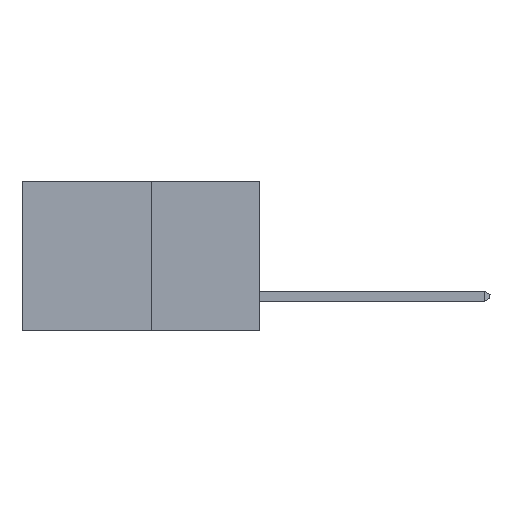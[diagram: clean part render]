
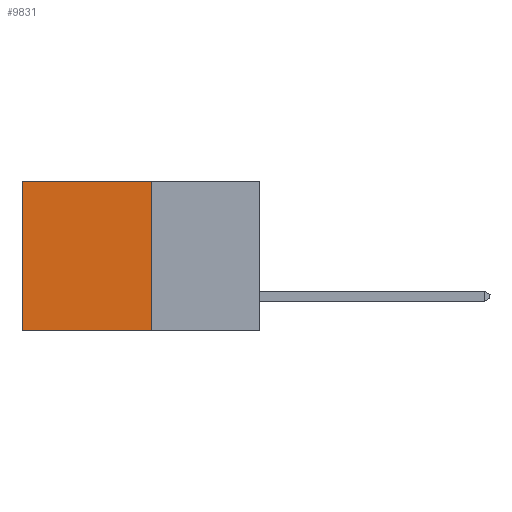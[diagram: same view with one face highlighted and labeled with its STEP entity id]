
A CAD part, left-side view. The second image highlights one B-rep face of the part: STEP entity #9831.
In plain terms, the highlighted planar face has unit normal (-1, 0, 0).
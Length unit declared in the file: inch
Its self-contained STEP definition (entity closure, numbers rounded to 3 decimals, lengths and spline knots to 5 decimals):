
#175 = PLANE ( 'NONE',  #7219 ) ;
#224 = EDGE_CURVE ( 'NONE', #5719, #2187, #7277, .T. ) ;
#442 = EDGE_CURVE ( 'NONE', #2187, #12836, #11072, .T. ) ;
#1648 = CARTESIAN_POINT ( 'NONE',  ( 0.277, 0.59, 0. ) ) ;
#1807 = EDGE_CURVE ( 'NONE', #11247, #12836, #8447, .T. ) ;
#2187 = VERTEX_POINT ( 'NONE', #1648 ) ;
#2620 = DIRECTION ( 'NONE',  ( 0., 0., -1. ) ) ;
#2775 = DIRECTION ( 'NONE',  ( 0., 0., -1. ) ) ;
#2966 = EDGE_CURVE ( 'NONE', #5719, #11247, #7939, .T. ) ;
#4893 = CARTESIAN_POINT ( 'NONE',  ( 0.277, 0.27, 0. ) ) ;
#5219 = DIRECTION ( 'NONE',  ( 0., 1., 0. ) ) ;
#5719 = VERTEX_POINT ( 'NONE', #4893 ) ;
#5843 = CARTESIAN_POINT ( 'NONE',  ( 0.277, 0.27, -0.37 ) ) ;
#6301 = FACE_OUTER_BOUND ( 'NONE', #10616, .T. ) ;
#6534 = ORIENTED_EDGE ( 'NONE', *, *, #1807, .F. ) ;
#6781 = DIRECTION ( 'NONE',  ( 0., 0., -1. ) ) ;
#7014 = CARTESIAN_POINT ( 'NONE',  ( 0.277, 0.27, -0.37 ) ) ;
#7073 = ORIENTED_EDGE ( 'NONE', *, *, #2966, .F. ) ;
#7118 = ORIENTED_EDGE ( 'NONE', *, *, #224, .T. ) ;
#7219 = AXIS2_PLACEMENT_3D ( 'NONE', #8006, #8978, #2620 ) ;
#7277 = LINE ( 'NONE', #9451, #11656 ) ;
#7328 = ORIENTED_EDGE ( 'NONE', *, *, #442, .T. ) ;
#7939 = LINE ( 'NONE', #7014, #12591 ) ;
#8006 = CARTESIAN_POINT ( 'NONE',  ( 0.277, 0.27, -0.37 ) ) ;
#8055 = DIRECTION ( 'NONE',  ( 0., 1., 0. ) ) ;
#8203 = CARTESIAN_POINT ( 'NONE',  ( 0.277, 0.59, -0.37 ) ) ;
#8447 = LINE ( 'NONE', #5843, #10629 ) ;
#8629 = VECTOR ( 'NONE', #6781, 39.37008 ) ;
#8724 = CARTESIAN_POINT ( 'NONE',  ( 0.277, 0.27, -0.37 ) ) ;
#8978 = DIRECTION ( 'NONE',  ( 1., 0., 0. ) ) ;
#9156 = CARTESIAN_POINT ( 'NONE',  ( 0.277, 0.59, -0.37 ) ) ;
#9451 = CARTESIAN_POINT ( 'NONE',  ( 0.277, 0.27, 0. ) ) ;
#9831 = ADVANCED_FACE ( 'NONE', ( #6301 ), #175, .F. ) ;
#10616 = EDGE_LOOP ( 'NONE', ( #7328, #6534, #7073, #7118 ) ) ;
#10629 = VECTOR ( 'NONE', #5219, 39.37008 ) ;
#11072 = LINE ( 'NONE', #9156, #8629 ) ;
#11247 = VERTEX_POINT ( 'NONE', #8724 ) ;
#11656 = VECTOR ( 'NONE', #8055, 39.37008 ) ;
#12591 = VECTOR ( 'NONE', #2775, 39.37008 ) ;
#12836 = VERTEX_POINT ( 'NONE', #8203 ) ;
